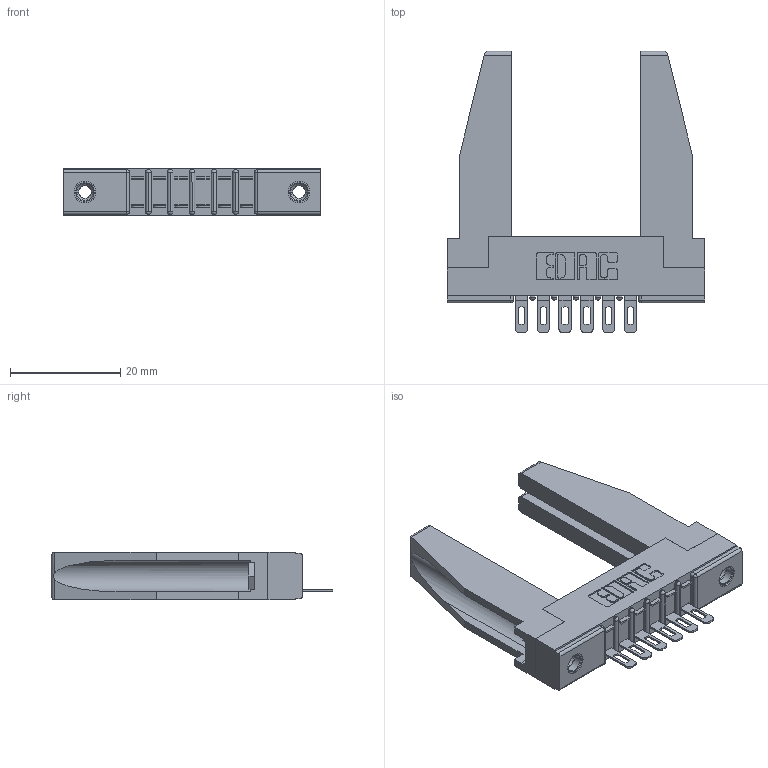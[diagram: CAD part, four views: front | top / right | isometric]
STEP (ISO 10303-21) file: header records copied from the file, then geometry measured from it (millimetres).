
FILE_DESCRIPTION (( 'STEP AP203' ), '1' );
FILE_NAME ('307-006-401-178.STEP', '2020-09-25T00:34:14', ( '' ), ( '' ), 'SwSTEP 2.0', 'SolidWorks 2020', '' );
FILE_SCHEMA (( 'CONFIG_CONTROL_DESIGN' ));
Length unit declared in the file: inch
Products named in the file (5): 307-220-078; 307 Part_.156 Dia Mounting Holes; 307-290-002_501; 307-006-401-178; 345-250-001_345-250-001-102
Assembly tree (11 placements, depth 2):
  307-006-401-178
    307 Part_.156 Dia Mounting Holes
    307-290-002_501  x6
    307-220-078  x2
    345-250-001_345-250-001-102  x2
Bounding box: 46.79 x 51.13 x 8.71 mm (x, y, z)
Volume: 7079 mm3; surface area: 8583.7 mm2
Topology: 11 solids, 11 shells, 711 faces, 2081 edges, 1358 vertices
Faces by surface type: plane 418, cylinder 263, sphere 14, cone 12, torus 4
Entity records: 12815 total; most frequent: CARTESIAN_POINT 2154, ORIENTED_EDGE 2100, DIRECTION 2070, EDGE_CURVE 1050, LINE 786, VECTOR 786, VERTEX_POINT 684, AXIS2_PLACEMENT_3D 642
